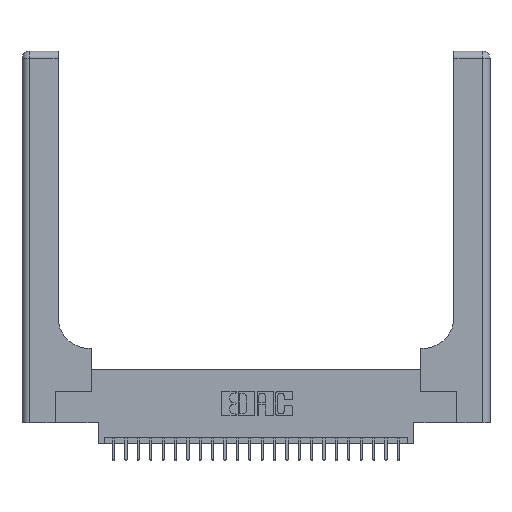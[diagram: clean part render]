
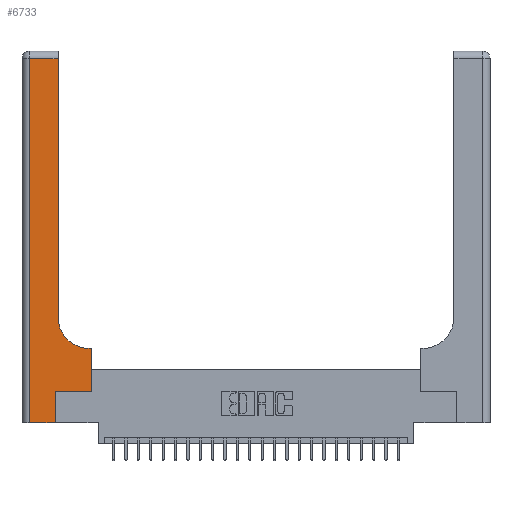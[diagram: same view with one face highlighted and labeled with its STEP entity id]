
A CAD part, top view. The second image highlights one B-rep face of the part: STEP entity #6733.
In plain terms, the highlighted planar face has unit normal (0, 0, 1).
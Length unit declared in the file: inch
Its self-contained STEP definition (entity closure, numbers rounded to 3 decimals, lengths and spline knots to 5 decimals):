
#372 = EDGE_CURVE ( 'NONE', #19838, #22920, #17979, .T. ) ;
#786 = DIRECTION ( 'NONE',  ( 1., 0., 0. ) ) ;
#1106 = ORIENTED_EDGE ( 'NONE', *, *, #23836, .T. ) ;
#1452 = LINE ( 'NONE', #1714, #19480 ) ;
#1606 = LINE ( 'NONE', #20302, #20374 ) ;
#1714 = CARTESIAN_POINT ( 'NONE',  ( 0., 2.94, 0.37 ) ) ;
#2015 = LINE ( 'NONE', #26335, #14305 ) ;
#2196 = CARTESIAN_POINT ( 'NONE',  ( 0.5585, 0.25, 0.37 ) ) ;
#3362 = CARTESIAN_POINT ( 'NONE',  ( 0.2915, 0.85, 0.37 ) ) ;
#3950 = ORIENTED_EDGE ( 'NONE', *, *, #22878, .T. ) ;
#4338 = CARTESIAN_POINT ( 'NONE',  ( 0.5585, 0.25, 0.37 ) ) ;
#4640 = DIRECTION ( 'NONE',  ( 1., 0., 0. ) ) ;
#4739 = ORIENTED_EDGE ( 'NONE', *, *, #23641, .T. ) ;
#5152 = VERTEX_POINT ( 'NONE', #5646 ) ;
#5646 = CARTESIAN_POINT ( 'NONE',  ( 0.5585, 0.6, 0.37 ) ) ;
#6043 = DIRECTION ( 'NONE',  ( -1., 0., 0. ) ) ;
#6167 = EDGE_CURVE ( 'NONE', #13471, #16926, #18625, .T. ) ;
#6733 = ADVANCED_FACE ( 'NONE', ( #22572 ), #12809, .F. ) ;
#7072 = AXIS2_PLACEMENT_3D ( 'NONE', #24581, #20958, #6043 ) ;
#7678 = VECTOR ( 'NONE', #16836, 39.37008 ) ;
#7683 = ORIENTED_EDGE ( 'NONE', *, *, #14946, .T. ) ;
#7767 = ORIENTED_EDGE ( 'NONE', *, *, #6167, .T. ) ;
#7834 = DIRECTION ( 'NONE',  ( -1., 0., 0. ) ) ;
#7879 = EDGE_CURVE ( 'NONE', #14907, #19838, #10641, .T. ) ;
#8050 = ORIENTED_EDGE ( 'NONE', *, *, #372, .T. ) ;
#8249 = DIRECTION ( 'NONE',  ( 0., -1., 0. ) ) ;
#9874 = VERTEX_POINT ( 'NONE', #4338 ) ;
#10117 = CARTESIAN_POINT ( 'NONE',  ( 0.2915, 3., 0.37 ) ) ;
#10448 = DIRECTION ( 'NONE',  ( 0., 1., 0. ) ) ;
#10641 = CIRCLE ( 'NONE', #25725, 0.25 ) ;
#10934 = DIRECTION ( 'NONE',  ( 0., 0., -1. ) ) ;
#11030 = CARTESIAN_POINT ( 'NONE',  ( 0.06, 0., 0.37 ) ) ;
#12194 = ORIENTED_EDGE ( 'NONE', *, *, #14929, .T. ) ;
#12627 = CARTESIAN_POINT ( 'NONE',  ( 0., 0., 0.37 ) ) ;
#12809 = PLANE ( 'NONE',  #7072 ) ;
#13033 = CARTESIAN_POINT ( 'NONE',  ( 0.269, 0.25, 0.37 ) ) ;
#13407 = CARTESIAN_POINT ( 'NONE',  ( 0.2915, 2.94, 0.37 ) ) ;
#13471 = VERTEX_POINT ( 'NONE', #11030 ) ;
#13726 = VECTOR ( 'NONE', #24186, 39.37008 ) ;
#14268 = EDGE_CURVE ( 'NONE', #22920, #21034, #1452, .T. ) ;
#14305 = VECTOR ( 'NONE', #8249, 39.37008 ) ;
#14907 = VERTEX_POINT ( 'NONE', #15832 ) ;
#14929 = EDGE_CURVE ( 'NONE', #5152, #14907, #1606, .T. ) ;
#14946 = EDGE_CURVE ( 'NONE', #21034, #13471, #2015, .T. ) ;
#15209 = LINE ( 'NONE', #13033, #25356 ) ;
#15316 = CARTESIAN_POINT ( 'NONE',  ( 0.269, 0., 0.37 ) ) ;
#15445 = LINE ( 'NONE', #15316, #23612 ) ;
#15832 = CARTESIAN_POINT ( 'NONE',  ( 0.5415, 0.6, 0.37 ) ) ;
#15874 = VECTOR ( 'NONE', #10448, 39.37008 ) ;
#16172 = CARTESIAN_POINT ( 'NONE',  ( 0.269, 0.25, 0.37 ) ) ;
#16836 = DIRECTION ( 'NONE',  ( 1., 0., 0. ) ) ;
#16926 = VERTEX_POINT ( 'NONE', #26341 ) ;
#17979 = LINE ( 'NONE', #10117, #13726 ) ;
#18096 = DIRECTION ( 'NONE',  ( -1., 0., 0. ) ) ;
#18446 = LINE ( 'NONE', #2196, #15874 ) ;
#18625 = LINE ( 'NONE', #12627, #7678 ) ;
#19037 = EDGE_LOOP ( 'NONE', ( #8050, #25886, #7683, #7767, #3950, #4739, #1106, #12194, #24084 ) ) ;
#19480 = VECTOR ( 'NONE', #18096, 39.37008 ) ;
#19737 = CARTESIAN_POINT ( 'NONE',  ( 0.5415, 0.85, 0.37 ) ) ;
#19784 = CARTESIAN_POINT ( 'NONE',  ( 0.06, 2.94, 0.37 ) ) ;
#19838 = VERTEX_POINT ( 'NONE', #3362 ) ;
#20302 = CARTESIAN_POINT ( 'NONE',  ( 0.2915, 0.6, 0.37 ) ) ;
#20374 = VECTOR ( 'NONE', #7834, 39.37008 ) ;
#20958 = DIRECTION ( 'NONE',  ( 0., 0., -1. ) ) ;
#21034 = VERTEX_POINT ( 'NONE', #19784 ) ;
#21808 = VERTEX_POINT ( 'NONE', #16172 ) ;
#22572 = FACE_OUTER_BOUND ( 'NONE', #19037, .T. ) ;
#22878 = EDGE_CURVE ( 'NONE', #16926, #21808, #15445, .T. ) ;
#22920 = VERTEX_POINT ( 'NONE', #13407 ) ;
#23566 = DIRECTION ( 'NONE',  ( 0., 1., 0. ) ) ;
#23612 = VECTOR ( 'NONE', #23566, 39.37008 ) ;
#23641 = EDGE_CURVE ( 'NONE', #21808, #9874, #15209, .T. ) ;
#23836 = EDGE_CURVE ( 'NONE', #9874, #5152, #18446, .T. ) ;
#24084 = ORIENTED_EDGE ( 'NONE', *, *, #7879, .T. ) ;
#24186 = DIRECTION ( 'NONE',  ( 0., 1., 0. ) ) ;
#24581 = CARTESIAN_POINT ( 'NONE',  ( 0., 3., 0.37 ) ) ;
#25356 = VECTOR ( 'NONE', #4640, 39.37008 ) ;
#25725 = AXIS2_PLACEMENT_3D ( 'NONE', #19737, #10934, #786 ) ;
#25886 = ORIENTED_EDGE ( 'NONE', *, *, #14268, .T. ) ;
#26335 = CARTESIAN_POINT ( 'NONE',  ( 0.06, 3., 0.37 ) ) ;
#26341 = CARTESIAN_POINT ( 'NONE',  ( 0.269, 0., 0.37 ) ) ;
